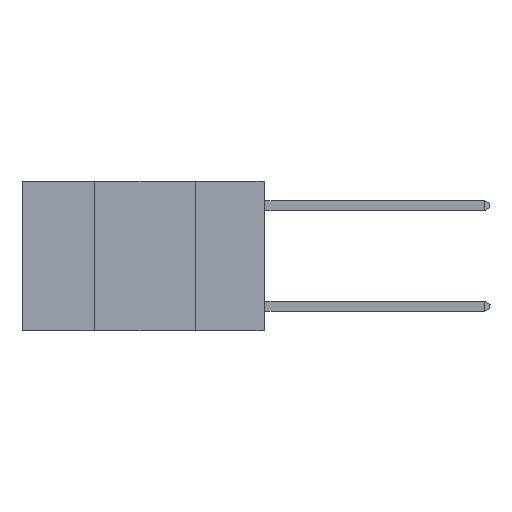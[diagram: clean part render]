
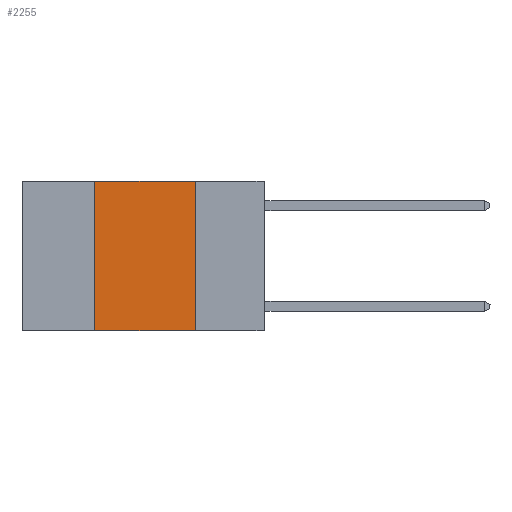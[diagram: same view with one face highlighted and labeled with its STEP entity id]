
A CAD part, left-side view. The second image highlights one B-rep face of the part: STEP entity #2255.
In plain terms, the highlighted planar face has unit normal (-1, 0, 0).
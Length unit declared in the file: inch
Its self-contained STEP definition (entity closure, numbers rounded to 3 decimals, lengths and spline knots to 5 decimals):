
#335 = VERTEX_POINT ( 'NONE', #9205 ) ;
#399 = LINE ( 'NONE', #4907, #2406 ) ;
#440 = DIRECTION ( 'NONE',  ( 0., 0., -1. ) ) ;
#454 = DIRECTION ( 'NONE',  ( 1., 0., 0. ) ) ;
#474 = CARTESIAN_POINT ( 'NONE',  ( 0., 0.6, 0. ) ) ;
#485 = PLANE ( 'NONE',  #4393 ) ;
#532 = LINE ( 'NONE', #4576, #7205 ) ;
#1543 = VERTEX_POINT ( 'NONE', #3665 ) ;
#1859 = LINE ( 'NONE', #2679, #8844 ) ;
#1993 = ORIENTED_EDGE ( 'NONE', *, *, #5558, .T. ) ;
#2255 = ADVANCED_FACE ( 'NONE', ( #8126 ), #485, .F. ) ;
#2406 = VECTOR ( 'NONE', #5790, 39.37008 ) ;
#2679 = CARTESIAN_POINT ( 'NONE',  ( 0., 0.6, 0. ) ) ;
#3068 = ORIENTED_EDGE ( 'NONE', *, *, #5736, .F. ) ;
#3310 = CARTESIAN_POINT ( 'NONE',  ( 0., 0.42, 0. ) ) ;
#3314 = LINE ( 'NONE', #9688, #9966 ) ;
#3568 = DIRECTION ( 'NONE',  ( 0., 0., -1. ) ) ;
#3665 = CARTESIAN_POINT ( 'NONE',  ( 0., 0.17, -0.37 ) ) ;
#4393 = AXIS2_PLACEMENT_3D ( 'NONE', #474, #454, #440 ) ;
#4541 = CARTESIAN_POINT ( 'NONE',  ( 0., 0.42, -0.37 ) ) ;
#4576 = CARTESIAN_POINT ( 'NONE',  ( 0., 0.6, -0.37 ) ) ;
#4836 = VERTEX_POINT ( 'NONE', #3310 ) ;
#4907 = CARTESIAN_POINT ( 'NONE',  ( 0., 0.42, 0. ) ) ;
#5449 = EDGE_CURVE ( 'NONE', #4836, #335, #1859, .T. ) ;
#5484 = EDGE_CURVE ( 'NONE', #335, #1543, #3314, .T. ) ;
#5558 = EDGE_CURVE ( 'NONE', #7771, #1543, #532, .T. ) ;
#5736 = EDGE_CURVE ( 'NONE', #7771, #4836, #399, .T. ) ;
#5790 = DIRECTION ( 'NONE',  ( 0., 0., 1. ) ) ;
#6048 = ORIENTED_EDGE ( 'NONE', *, *, #5449, .F. ) ;
#6065 = ORIENTED_EDGE ( 'NONE', *, *, #5484, .F. ) ;
#7091 = DIRECTION ( 'NONE',  ( 0., -1., 0. ) ) ;
#7205 = VECTOR ( 'NONE', #8160, 39.37008 ) ;
#7771 = VERTEX_POINT ( 'NONE', #4541 ) ;
#8126 = FACE_OUTER_BOUND ( 'NONE', #9248, .T. ) ;
#8160 = DIRECTION ( 'NONE',  ( 0., -1., 0. ) ) ;
#8844 = VECTOR ( 'NONE', #7091, 39.37008 ) ;
#9205 = CARTESIAN_POINT ( 'NONE',  ( 0., 0.17, 0. ) ) ;
#9248 = EDGE_LOOP ( 'NONE', ( #6065, #6048, #3068, #1993 ) ) ;
#9688 = CARTESIAN_POINT ( 'NONE',  ( 0., 0.17, 0. ) ) ;
#9966 = VECTOR ( 'NONE', #3568, 39.37008 ) ;
